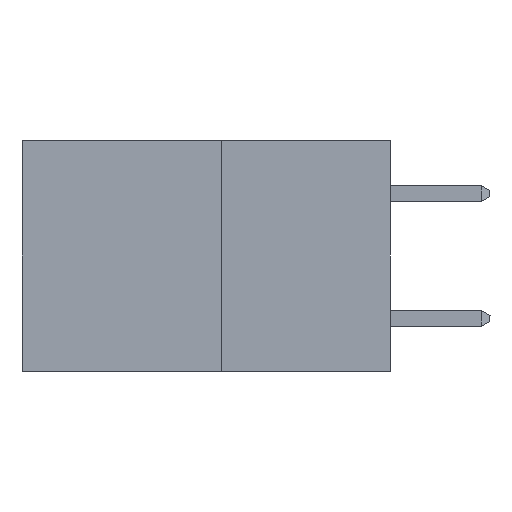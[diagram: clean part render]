
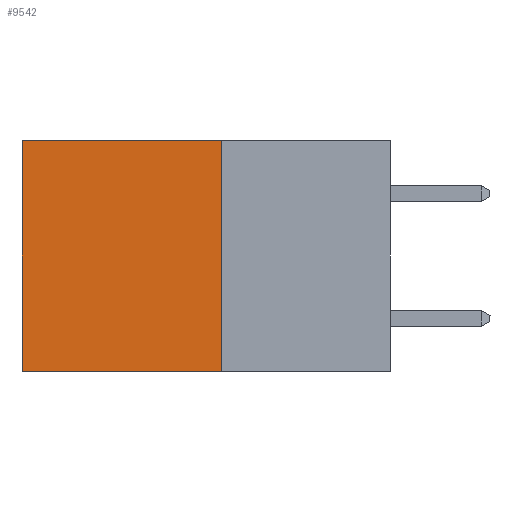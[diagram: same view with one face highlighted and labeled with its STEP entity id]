
A CAD part, left-side view. The second image highlights one B-rep face of the part: STEP entity #9542.
In plain terms, the highlighted planar face has unit normal (-1, 0, 0).
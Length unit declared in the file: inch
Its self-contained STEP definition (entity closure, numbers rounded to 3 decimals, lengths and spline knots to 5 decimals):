
#670 = AXIS2_PLACEMENT_3D ( 'NONE', #13442, #721, #8066 ) ;
#721 = DIRECTION ( 'NONE',  ( 1., 0., 0. ) ) ;
#725 = VERTEX_POINT ( 'NONE', #1524 ) ;
#1272 = VECTOR ( 'NONE', #5118, 39.37008 ) ;
#1524 = CARTESIAN_POINT ( 'NONE',  ( 0.277, 0.27, 0. ) ) ;
#1993 = CARTESIAN_POINT ( 'NONE',  ( 0.277, 0.27, -0.37 ) ) ;
#3413 = ORIENTED_EDGE ( 'NONE', *, *, #7944, .F. ) ;
#3420 = FACE_OUTER_BOUND ( 'NONE', #11740, .T. ) ;
#3859 = VECTOR ( 'NONE', #8812, 39.37008 ) ;
#4523 = VERTEX_POINT ( 'NONE', #9342 ) ;
#4575 = VERTEX_POINT ( 'NONE', #9037 ) ;
#4613 = EDGE_CURVE ( 'NONE', #9415, #4575, #13207, .T. ) ;
#5070 = VECTOR ( 'NONE', #13565, 39.37008 ) ;
#5118 = DIRECTION ( 'NONE',  ( 0., 1., 0. ) ) ;
#5346 = EDGE_CURVE ( 'NONE', #725, #9415, #12375, .T. ) ;
#5395 = LINE ( 'NONE', #12516, #5070 ) ;
#6331 = ORIENTED_EDGE ( 'NONE', *, *, #4613, .T. ) ;
#6549 = DIRECTION ( 'NONE',  ( 0., 0., -1. ) ) ;
#7140 = CARTESIAN_POINT ( 'NONE',  ( 0.277, 0.59, -0.37 ) ) ;
#7768 = ORIENTED_EDGE ( 'NONE', *, *, #11121, .F. ) ;
#7944 = EDGE_CURVE ( 'NONE', #725, #4523, #5395, .T. ) ;
#8066 = DIRECTION ( 'NONE',  ( 0., 0., -1. ) ) ;
#8764 = CARTESIAN_POINT ( 'NONE',  ( 0.277, 0.27, 0. ) ) ;
#8812 = DIRECTION ( 'NONE',  ( 0., 1., 0. ) ) ;
#9022 = ORIENTED_EDGE ( 'NONE', *, *, #5346, .T. ) ;
#9037 = CARTESIAN_POINT ( 'NONE',  ( 0.277, 0.59, -0.37 ) ) ;
#9342 = CARTESIAN_POINT ( 'NONE',  ( 0.277, 0.27, -0.37 ) ) ;
#9415 = VERTEX_POINT ( 'NONE', #13259 ) ;
#9542 = ADVANCED_FACE ( 'NONE', ( #3420 ), #12393, .F. ) ;
#10748 = LINE ( 'NONE', #1993, #1272 ) ;
#11121 = EDGE_CURVE ( 'NONE', #4523, #4575, #10748, .T. ) ;
#11740 = EDGE_LOOP ( 'NONE', ( #6331, #7768, #3413, #9022 ) ) ;
#12375 = LINE ( 'NONE', #8764, #3859 ) ;
#12393 = PLANE ( 'NONE',  #670 ) ;
#12516 = CARTESIAN_POINT ( 'NONE',  ( 0.277, 0.27, -0.37 ) ) ;
#12885 = VECTOR ( 'NONE', #6549, 39.37008 ) ;
#13207 = LINE ( 'NONE', #7140, #12885 ) ;
#13259 = CARTESIAN_POINT ( 'NONE',  ( 0.277, 0.59, 0. ) ) ;
#13442 = CARTESIAN_POINT ( 'NONE',  ( 0.277, 0.27, -0.37 ) ) ;
#13565 = DIRECTION ( 'NONE',  ( 0., 0., -1. ) ) ;
